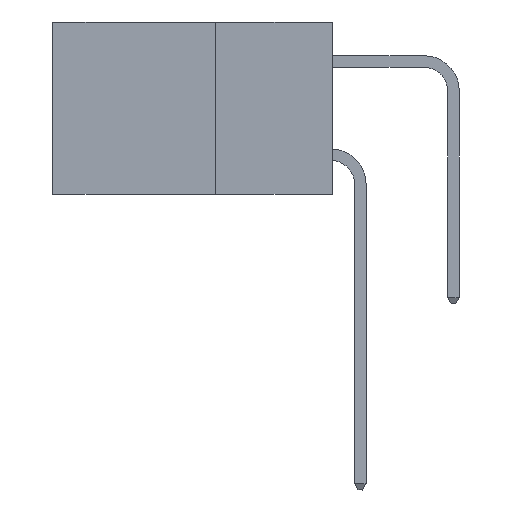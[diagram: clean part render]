
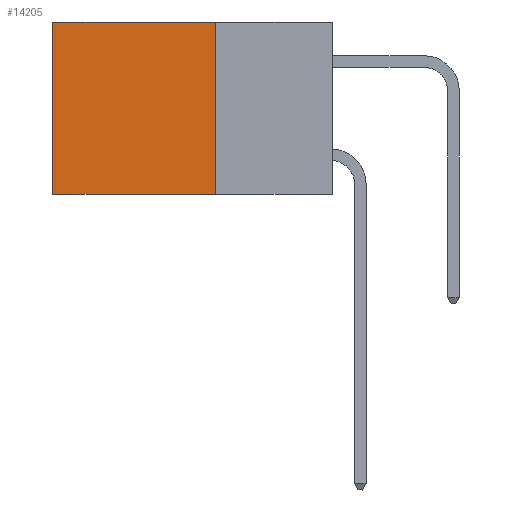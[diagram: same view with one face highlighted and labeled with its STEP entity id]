
A CAD part, left-side view. The second image highlights one B-rep face of the part: STEP entity #14205.
In plain terms, the highlighted planar face has unit normal (-1, 0, 0).
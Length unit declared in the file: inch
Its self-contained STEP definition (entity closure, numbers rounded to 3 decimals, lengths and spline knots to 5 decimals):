
#2234 = CARTESIAN_POINT ( 'NONE',  ( 0.298, 0.25, 0. ) ) ;
#2862 = LINE ( 'NONE', #14004, #19980 ) ;
#2920 = CARTESIAN_POINT ( 'NONE',  ( 0.298, 0.25, -0.37 ) ) ;
#4453 = DIRECTION ( 'NONE',  ( 0., 0., -1. ) ) ;
#5068 = LINE ( 'NONE', #2234, #19890 ) ;
#5462 = DIRECTION ( 'NONE',  ( 0., 1., 0. ) ) ;
#5679 = CARTESIAN_POINT ( 'NONE',  ( 0.298, 0.6, -0.37 ) ) ;
#5905 = ORIENTED_EDGE ( 'NONE', *, *, #13029, .T. ) ;
#7569 = CARTESIAN_POINT ( 'NONE',  ( 0.298, 0.25, 0. ) ) ;
#7863 = EDGE_CURVE ( 'NONE', #21468, #10867, #20738, .T. ) ;
#7988 = FACE_OUTER_BOUND ( 'NONE', #22296, .T. ) ;
#8225 = ORIENTED_EDGE ( 'NONE', *, *, #25826, .F. ) ;
#10867 = VERTEX_POINT ( 'NONE', #5679 ) ;
#10910 = CARTESIAN_POINT ( 'NONE',  ( 0.298, 0.6, 0. ) ) ;
#11553 = DIRECTION ( 'NONE',  ( 1., 0., 0. ) ) ;
#12607 = VERTEX_POINT ( 'NONE', #2920 ) ;
#13029 = EDGE_CURVE ( 'NONE', #25095, #21468, #2862, .T. ) ;
#14004 = CARTESIAN_POINT ( 'NONE',  ( 0.298, 0.25, 0. ) ) ;
#14205 = ADVANCED_FACE ( 'NONE', ( #7988 ), #17991, .F. ) ;
#14853 = VECTOR ( 'NONE', #16977, 39.37008 ) ;
#16221 = CARTESIAN_POINT ( 'NONE',  ( 0.298, 0.25, -0.37 ) ) ;
#16977 = DIRECTION ( 'NONE',  ( 0., 0., -1. ) ) ;
#17507 = CARTESIAN_POINT ( 'NONE',  ( 0.298, 0.6, 0. ) ) ;
#17762 = AXIS2_PLACEMENT_3D ( 'NONE', #7569, #11553, #26260 ) ;
#17991 = PLANE ( 'NONE',  #17762 ) ;
#18329 = DIRECTION ( 'NONE',  ( 0., 1., 0. ) ) ;
#19890 = VECTOR ( 'NONE', #4453, 39.37008 ) ;
#19980 = VECTOR ( 'NONE', #5462, 39.37008 ) ;
#20309 = CARTESIAN_POINT ( 'NONE',  ( 0.298, 0.25, 0. ) ) ;
#20433 = ORIENTED_EDGE ( 'NONE', *, *, #7863, .T. ) ;
#20738 = LINE ( 'NONE', #10910, #14853 ) ;
#21468 = VERTEX_POINT ( 'NONE', #17507 ) ;
#22296 = EDGE_LOOP ( 'NONE', ( #20433, #8225, #24504, #5905 ) ) ;
#23252 = EDGE_CURVE ( 'NONE', #25095, #12607, #5068, .T. ) ;
#23919 = VECTOR ( 'NONE', #18329, 39.37008 ) ;
#24504 = ORIENTED_EDGE ( 'NONE', *, *, #23252, .F. ) ;
#25095 = VERTEX_POINT ( 'NONE', #20309 ) ;
#25826 = EDGE_CURVE ( 'NONE', #12607, #10867, #26859, .T. ) ;
#26260 = DIRECTION ( 'NONE',  ( 0., 0., -1. ) ) ;
#26859 = LINE ( 'NONE', #16221, #23919 ) ;
